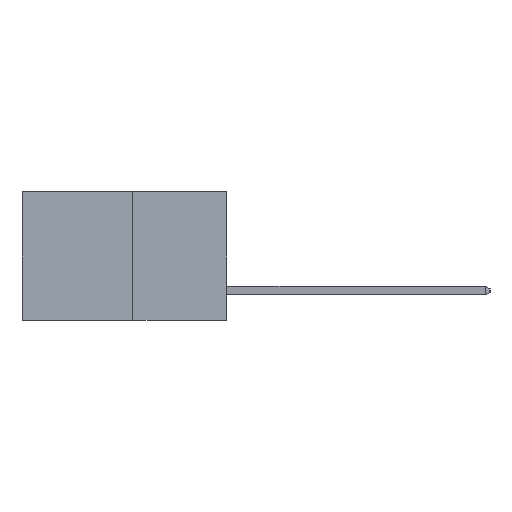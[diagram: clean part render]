
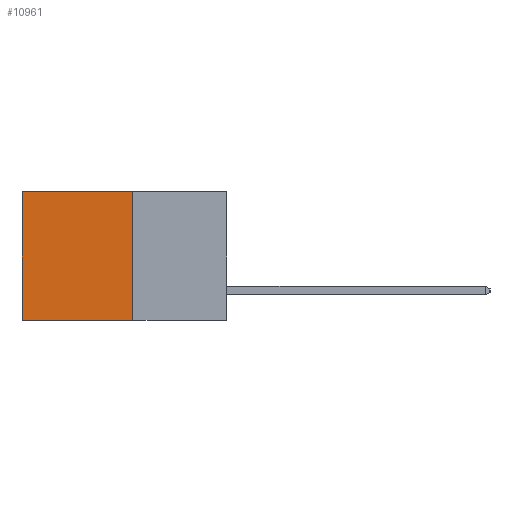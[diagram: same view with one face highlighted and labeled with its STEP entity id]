
A CAD part, left-side view. The second image highlights one B-rep face of the part: STEP entity #10961.
In plain terms, the highlighted planar face has unit normal (-1, 0, 0).
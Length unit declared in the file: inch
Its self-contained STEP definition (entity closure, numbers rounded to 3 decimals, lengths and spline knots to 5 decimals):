
#288 = VERTEX_POINT ( 'NONE', #7543 ) ;
#301 = LINE ( 'NONE', #10559, #7142 ) ;
#457 = AXIS2_PLACEMENT_3D ( 'NONE', #6094, #2622, #8538 ) ;
#570 = EDGE_CURVE ( 'NONE', #8508, #1883, #3540, .T. ) ;
#712 = VECTOR ( 'NONE', #1448, 39.37008 ) ;
#1320 = EDGE_CURVE ( 'NONE', #288, #3496, #2060, .T. ) ;
#1448 = DIRECTION ( 'NONE',  ( 0., 0., -1. ) ) ;
#1449 = CARTESIAN_POINT ( 'NONE',  ( 0.277, 0.27, -0.37 ) ) ;
#1883 = VERTEX_POINT ( 'NONE', #5170 ) ;
#2060 = LINE ( 'NONE', #6061, #5296 ) ;
#2622 = DIRECTION ( 'NONE',  ( 1., 0., 0. ) ) ;
#2985 = CARTESIAN_POINT ( 'NONE',  ( 0.277, 0.27, -0.37 ) ) ;
#3251 = CARTESIAN_POINT ( 'NONE',  ( 0.277, 0.27, -0.37 ) ) ;
#3262 = LINE ( 'NONE', #1449, #712 ) ;
#3496 = VERTEX_POINT ( 'NONE', #4748 ) ;
#3540 = LINE ( 'NONE', #2985, #7724 ) ;
#3640 = ORIENTED_EDGE ( 'NONE', *, *, #4114, .T. ) ;
#3727 = ORIENTED_EDGE ( 'NONE', *, *, #570, .F. ) ;
#3742 = ORIENTED_EDGE ( 'NONE', *, *, #6989, .F. ) ;
#3798 = EDGE_LOOP ( 'NONE', ( #3640, #3727, #3742, #3910 ) ) ;
#3910 = ORIENTED_EDGE ( 'NONE', *, *, #1320, .T. ) ;
#4114 = EDGE_CURVE ( 'NONE', #3496, #1883, #301, .T. ) ;
#4748 = CARTESIAN_POINT ( 'NONE',  ( 0.277, 0.59, 0. ) ) ;
#5170 = CARTESIAN_POINT ( 'NONE',  ( 0.277, 0.59, -0.37 ) ) ;
#5296 = VECTOR ( 'NONE', #8548, 39.37008 ) ;
#6061 = CARTESIAN_POINT ( 'NONE',  ( 0.277, 0.27, 0. ) ) ;
#6094 = CARTESIAN_POINT ( 'NONE',  ( 0.277, 0.27, -0.37 ) ) ;
#6122 = FACE_OUTER_BOUND ( 'NONE', #3798, .T. ) ;
#6907 = PLANE ( 'NONE',  #457 ) ;
#6989 = EDGE_CURVE ( 'NONE', #288, #8508, #3262, .T. ) ;
#7142 = VECTOR ( 'NONE', #10503, 39.37008 ) ;
#7543 = CARTESIAN_POINT ( 'NONE',  ( 0.277, 0.27, 0. ) ) ;
#7724 = VECTOR ( 'NONE', #8501, 39.37008 ) ;
#8501 = DIRECTION ( 'NONE',  ( 0., 1., 0. ) ) ;
#8508 = VERTEX_POINT ( 'NONE', #3251 ) ;
#8538 = DIRECTION ( 'NONE',  ( 0., 0., -1. ) ) ;
#8548 = DIRECTION ( 'NONE',  ( 0., 1., 0. ) ) ;
#10503 = DIRECTION ( 'NONE',  ( 0., 0., -1. ) ) ;
#10559 = CARTESIAN_POINT ( 'NONE',  ( 0.277, 0.59, -0.37 ) ) ;
#10961 = ADVANCED_FACE ( 'NONE', ( #6122 ), #6907, .F. ) ;
